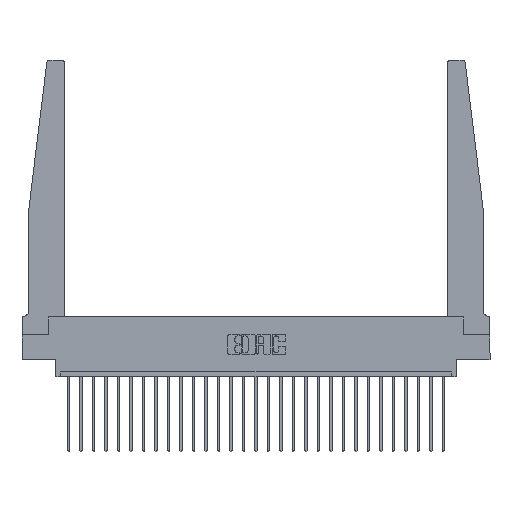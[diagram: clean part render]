
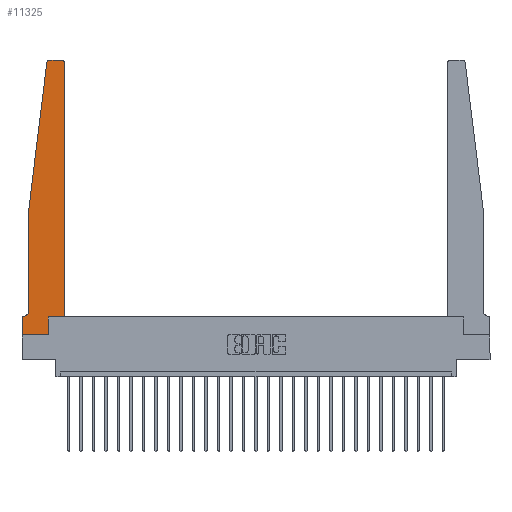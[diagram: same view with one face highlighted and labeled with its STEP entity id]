
A CAD part, top view. The second image highlights one B-rep face of the part: STEP entity #11325.
In plain terms, the highlighted planar face has unit normal (0, 0, 1).
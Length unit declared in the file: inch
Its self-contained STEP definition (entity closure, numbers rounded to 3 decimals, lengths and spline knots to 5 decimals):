
#243 = AXIS2_PLACEMENT_3D ( 'NONE', #19617, #13793, #2108 ) ;
#558 = EDGE_CURVE ( 'NONE', #10616, #17127, #2564, .T. ) ;
#609 = DIRECTION ( 'NONE',  ( -1., 0., 0. ) ) ;
#1125 = VERTEX_POINT ( 'NONE', #18103 ) ;
#1527 = DIRECTION ( 'NONE',  ( 0., -1., 0. ) ) ;
#1837 = CARTESIAN_POINT ( 'NONE',  ( 0.425, 0.18, 0.37 ) ) ;
#2044 = VECTOR ( 'NONE', #19962, 39.37008 ) ;
#2108 = DIRECTION ( 'NONE',  ( 1., 0., 0. ) ) ;
#2227 = EDGE_CURVE ( 'NONE', #11753, #18894, #8078, .T. ) ;
#2238 = VECTOR ( 'NONE', #13749, 39.37008 ) ;
#2250 = VECTOR ( 'NONE', #7486, 39.37008 ) ;
#2353 = VECTOR ( 'NONE', #8380, 39.37008 ) ;
#2477 = ORIENTED_EDGE ( 'NONE', *, *, #8153, .T. ) ;
#2564 = LINE ( 'NONE', #9141, #7239 ) ;
#2689 = LINE ( 'NONE', #14112, #2044 ) ;
#2767 = CARTESIAN_POINT ( 'NONE',  ( 0.2605, 0.18, 0.37 ) ) ;
#2907 = ORIENTED_EDGE ( 'NONE', *, *, #2227, .T. ) ;
#3238 = VERTEX_POINT ( 'NONE', #14454 ) ;
#3526 = EDGE_CURVE ( 'NONE', #18894, #10616, #19945, .T. ) ;
#4216 = ORIENTED_EDGE ( 'NONE', *, *, #3526, .T. ) ;
#4319 = ORIENTED_EDGE ( 'NONE', *, *, #558, .T. ) ;
#4356 = VERTEX_POINT ( 'NONE', #13011 ) ;
#4397 = DIRECTION ( 'NONE',  ( 1., 0., 0. ) ) ;
#4698 = CARTESIAN_POINT ( 'NONE',  ( 0., 0., 0.37 ) ) ;
#5368 = DIRECTION ( 'NONE',  ( 0., 0., 1. ) ) ;
#6031 = CARTESIAN_POINT ( 'NONE',  ( 0.425, 2.72, 0.37 ) ) ;
#6415 = EDGE_CURVE ( 'NONE', #22501, #8236, #9933, .T. ) ;
#6490 = VERTEX_POINT ( 'NONE', #7522 ) ;
#6516 = CARTESIAN_POINT ( 'NONE',  ( 0.015, 0.2375, 0.37 ) ) ;
#6780 = DIRECTION ( 'NONE',  ( 0., 0., 1. ) ) ;
#7031 = CARTESIAN_POINT ( 'NONE',  ( 0.27653, 2.75, 0.37 ) ) ;
#7239 = VECTOR ( 'NONE', #10851, 39.37008 ) ;
#7486 = DIRECTION ( 'NONE',  ( 1., 0., 0. ) ) ;
#7522 = CARTESIAN_POINT ( 'NONE',  ( 0.015, 0.1875, 0.37 ) ) ;
#7548 = CARTESIAN_POINT ( 'NONE',  ( 0.25, 2.75, 0.37 ) ) ;
#7740 = CARTESIAN_POINT ( 'NONE',  ( 0.425, 0.18, 0.37 ) ) ;
#7773 = CARTESIAN_POINT ( 'NONE',  ( 0.24675, 2.72367, 0.37 ) ) ;
#7788 = EDGE_LOOP ( 'NONE', ( #16041, #23241, #19834, #16965, #10136, #12780, #21676, #2477, #2907, #4216, #4319, #23982 ) ) ;
#8040 = LINE ( 'NONE', #15276, #23178 ) ;
#8078 = LINE ( 'NONE', #2767, #23559 ) ;
#8153 = EDGE_CURVE ( 'NONE', #4356, #11753, #2689, .T. ) ;
#8236 = VERTEX_POINT ( 'NONE', #7773 ) ;
#8312 = EDGE_CURVE ( 'NONE', #17127, #9513, #24316, .T. ) ;
#8380 = DIRECTION ( 'NONE',  ( 0., -1., 0. ) ) ;
#8776 = CARTESIAN_POINT ( 'NONE',  ( 0.395, 2.75, 0.37 ) ) ;
#9141 = CARTESIAN_POINT ( 'NONE',  ( 0.425, 0.18, 0.37 ) ) ;
#9513 = VERTEX_POINT ( 'NONE', #8776 ) ;
#9933 = CIRCLE ( 'NONE', #22293, 0.03 ) ;
#10136 = ORIENTED_EDGE ( 'NONE', *, *, #19856, .T. ) ;
#10616 = VERTEX_POINT ( 'NONE', #1837 ) ;
#10851 = DIRECTION ( 'NONE',  ( 0., 1., 0. ) ) ;
#11071 = DIRECTION ( 'NONE',  ( 0., 0., -1. ) ) ;
#11325 = ADVANCED_FACE ( 'NONE', ( #19131 ), #14426, .T. ) ;
#11598 = LINE ( 'NONE', #21377, #2238 ) ;
#11753 = VERTEX_POINT ( 'NONE', #15478 ) ;
#11985 = CIRCLE ( 'NONE', #20237, 0.05 ) ;
#12267 = DIRECTION ( 'NONE',  ( -1., 0., 0. ) ) ;
#12705 = CARTESIAN_POINT ( 'NONE',  ( 0.065, 0.1875, 0.37 ) ) ;
#12780 = ORIENTED_EDGE ( 'NONE', *, *, #25140, .T. ) ;
#13011 = CARTESIAN_POINT ( 'NONE',  ( 0., 0., 0.37 ) ) ;
#13749 = DIRECTION ( 'NONE',  ( -0.122, -0.992, 0. ) ) ;
#13793 = DIRECTION ( 'NONE',  ( 0., 0., 1. ) ) ;
#13848 = AXIS2_PLACEMENT_3D ( 'NONE', #18643, #6780, #4397 ) ;
#14112 = CARTESIAN_POINT ( 'NONE',  ( 0., 0., 0.37 ) ) ;
#14426 = PLANE ( 'NONE',  #13848 ) ;
#14454 = CARTESIAN_POINT ( 'NONE',  ( 0.065, 0.2375, 0.37 ) ) ;
#14709 = EDGE_CURVE ( 'NONE', #8236, #18670, #11598, .T. ) ;
#14843 = DIRECTION ( 'NONE',  ( 0., 1., 0. ) ) ;
#15276 = CARTESIAN_POINT ( 'NONE',  ( 0.065, 1.25, 0.37 ) ) ;
#15354 = LINE ( 'NONE', #12705, #15987 ) ;
#15478 = CARTESIAN_POINT ( 'NONE',  ( 0.2605, 0., 0.37 ) ) ;
#15932 = VECTOR ( 'NONE', #21359, 39.37008 ) ;
#15987 = VECTOR ( 'NONE', #12267, 39.37008 ) ;
#16041 = ORIENTED_EDGE ( 'NONE', *, *, #21306, .T. ) ;
#16965 = ORIENTED_EDGE ( 'NONE', *, *, #22990, .T. ) ;
#17047 = CARTESIAN_POINT ( 'NONE',  ( 0.27653, 2.72, 0.37 ) ) ;
#17127 = VERTEX_POINT ( 'NONE', #6031 ) ;
#18103 = CARTESIAN_POINT ( 'NONE',  ( 0., 0.1875, 0.37 ) ) ;
#18643 = CARTESIAN_POINT ( 'NONE',  ( 0., 0.1875, 0.37 ) ) ;
#18670 = VERTEX_POINT ( 'NONE', #22376 ) ;
#18894 = VERTEX_POINT ( 'NONE', #25095 ) ;
#19131 = FACE_OUTER_BOUND ( 'NONE', #7788, .T. ) ;
#19230 = DIRECTION ( 'NONE',  ( 1., 0., 0. ) ) ;
#19617 = CARTESIAN_POINT ( 'NONE',  ( 0.395, 2.72, 0.37 ) ) ;
#19834 = ORIENTED_EDGE ( 'NONE', *, *, #14709, .T. ) ;
#19856 = EDGE_CURVE ( 'NONE', #3238, #6490, #11985, .T. ) ;
#19945 = LINE ( 'NONE', #7740, #2250 ) ;
#19962 = DIRECTION ( 'NONE',  ( 1., 0., 0. ) ) ;
#20237 = AXIS2_PLACEMENT_3D ( 'NONE', #6516, #11071, #609 ) ;
#20818 = LINE ( 'NONE', #7548, #15932 ) ;
#21306 = EDGE_CURVE ( 'NONE', #9513, #22501, #20818, .T. ) ;
#21359 = DIRECTION ( 'NONE',  ( -1., 0., 0. ) ) ;
#21377 = CARTESIAN_POINT ( 'NONE',  ( 0.065, 1.25, 0.37 ) ) ;
#21676 = ORIENTED_EDGE ( 'NONE', *, *, #23872, .T. ) ;
#22293 = AXIS2_PLACEMENT_3D ( 'NONE', #17047, #5368, #19230 ) ;
#22376 = CARTESIAN_POINT ( 'NONE',  ( 0.065, 1.25, 0.37 ) ) ;
#22501 = VERTEX_POINT ( 'NONE', #7031 ) ;
#22990 = EDGE_CURVE ( 'NONE', #18670, #3238, #8040, .T. ) ;
#23133 = LINE ( 'NONE', #4698, #2353 ) ;
#23178 = VECTOR ( 'NONE', #1527, 39.37008 ) ;
#23241 = ORIENTED_EDGE ( 'NONE', *, *, #6415, .T. ) ;
#23559 = VECTOR ( 'NONE', #14843, 39.37008 ) ;
#23872 = EDGE_CURVE ( 'NONE', #1125, #4356, #23133, .T. ) ;
#23982 = ORIENTED_EDGE ( 'NONE', *, *, #8312, .T. ) ;
#24316 = CIRCLE ( 'NONE', #243, 0.03 ) ;
#25095 = CARTESIAN_POINT ( 'NONE',  ( 0.2605, 0.18, 0.37 ) ) ;
#25140 = EDGE_CURVE ( 'NONE', #6490, #1125, #15354, .T. ) ;
